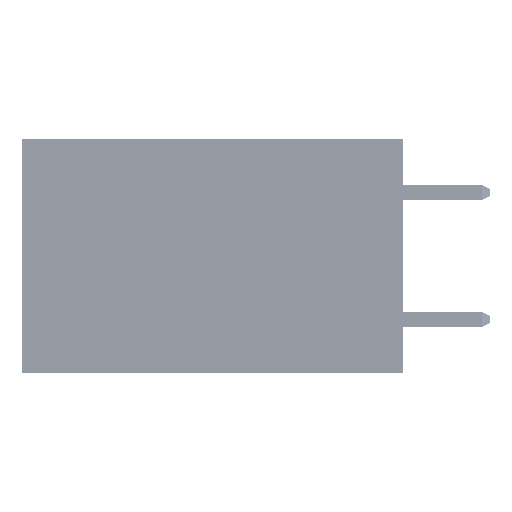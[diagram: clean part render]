
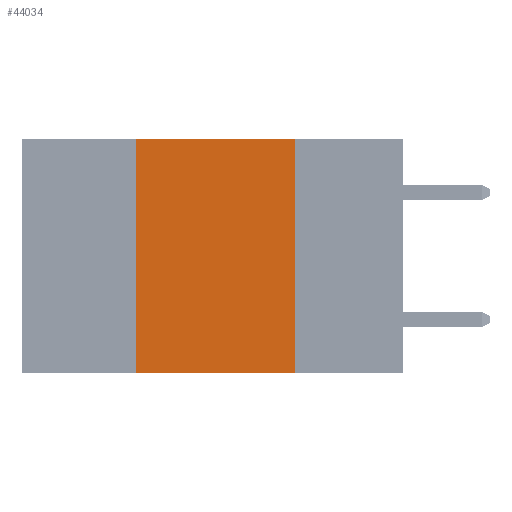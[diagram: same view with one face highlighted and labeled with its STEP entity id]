
A CAD part, left-side view. The second image highlights one B-rep face of the part: STEP entity #44034.
In plain terms, the highlighted planar face has unit normal (-1, 0, 0).
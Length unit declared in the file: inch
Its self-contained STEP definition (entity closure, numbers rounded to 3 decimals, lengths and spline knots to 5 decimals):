
#207 = DIRECTION ( 'NONE',  ( 0., 0., -1. ) ) ;
#226 = EDGE_CURVE ( 'NONE', #31395, #6316, #8604, .T. ) ;
#500 = VECTOR ( 'NONE', #36362, 39.37008 ) ;
#767 = FACE_OUTER_BOUND ( 'NONE', #14733, .T. ) ;
#6316 = VERTEX_POINT ( 'NONE', #38872 ) ;
#8604 = LINE ( 'NONE', #13862, #25110 ) ;
#8810 = LINE ( 'NONE', #27083, #39909 ) ;
#9212 = LINE ( 'NONE', #17679, #30080 ) ;
#11058 = EDGE_CURVE ( 'NONE', #17230, #6316, #8810, .T. ) ;
#12356 = DIRECTION ( 'NONE',  ( 1., 0., 0. ) ) ;
#13862 = CARTESIAN_POINT ( 'NONE',  ( 0., 0.6, -0.37 ) ) ;
#14733 = EDGE_LOOP ( 'NONE', ( #21370, #39105, #25482, #27589 ) ) ;
#17033 = CARTESIAN_POINT ( 'NONE',  ( 0., 0.42, -0.37 ) ) ;
#17230 = VERTEX_POINT ( 'NONE', #22013 ) ;
#17679 = CARTESIAN_POINT ( 'NONE',  ( 0., 0.42, 0. ) ) ;
#21370 = ORIENTED_EDGE ( 'NONE', *, *, #11058, .F. ) ;
#22013 = CARTESIAN_POINT ( 'NONE',  ( 0., 0.17, 0. ) ) ;
#24611 = CARTESIAN_POINT ( 'NONE',  ( 0., 0.6, 0. ) ) ;
#25110 = VECTOR ( 'NONE', #41111, 39.37008 ) ;
#25482 = ORIENTED_EDGE ( 'NONE', *, *, #30612, .F. ) ;
#27083 = CARTESIAN_POINT ( 'NONE',  ( 0., 0.17, 0. ) ) ;
#27172 = CARTESIAN_POINT ( 'NONE',  ( 0., 0.42, 0. ) ) ;
#27257 = DIRECTION ( 'NONE',  ( 0., 0., -1. ) ) ;
#27589 = ORIENTED_EDGE ( 'NONE', *, *, #226, .T. ) ;
#30080 = VECTOR ( 'NONE', #49085, 39.37008 ) ;
#30612 = EDGE_CURVE ( 'NONE', #31395, #33193, #9212, .T. ) ;
#31395 = VERTEX_POINT ( 'NONE', #17033 ) ;
#33193 = VERTEX_POINT ( 'NONE', #27172 ) ;
#35712 = CARTESIAN_POINT ( 'NONE',  ( 0., 0.6, 0. ) ) ;
#36362 = DIRECTION ( 'NONE',  ( 0., -1., 0. ) ) ;
#36548 = LINE ( 'NONE', #24611, #500 ) ;
#38872 = CARTESIAN_POINT ( 'NONE',  ( 0., 0.17, -0.37 ) ) ;
#39105 = ORIENTED_EDGE ( 'NONE', *, *, #41066, .F. ) ;
#39909 = VECTOR ( 'NONE', #27257, 39.37008 ) ;
#41066 = EDGE_CURVE ( 'NONE', #33193, #17230, #36548, .T. ) ;
#41111 = DIRECTION ( 'NONE',  ( 0., -1., 0. ) ) ;
#44034 = ADVANCED_FACE ( 'NONE', ( #767 ), #46978, .F. ) ;
#44403 = AXIS2_PLACEMENT_3D ( 'NONE', #35712, #12356, #207 ) ;
#46978 = PLANE ( 'NONE',  #44403 ) ;
#49085 = DIRECTION ( 'NONE',  ( 0., 0., 1. ) ) ;
